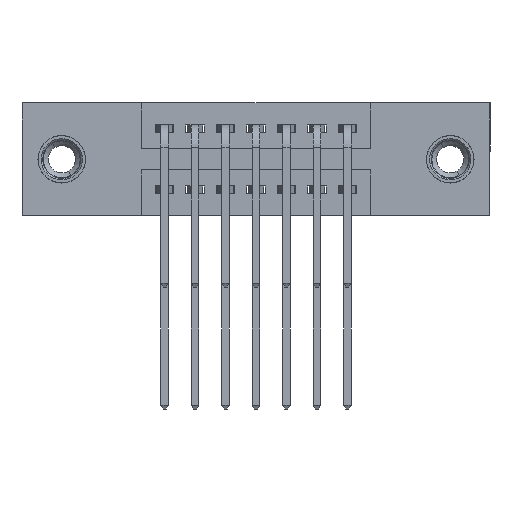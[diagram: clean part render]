
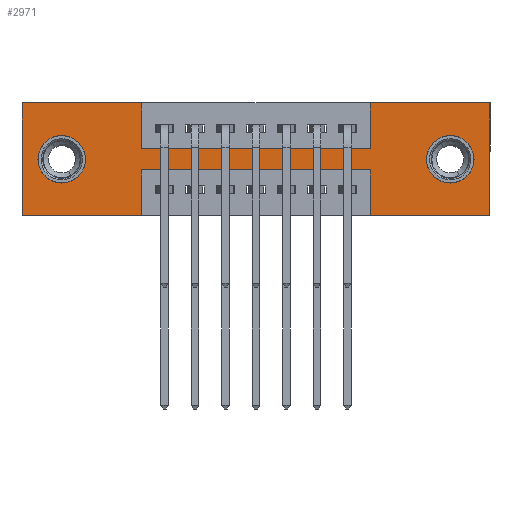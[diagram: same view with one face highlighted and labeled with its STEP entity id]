
A CAD part, front view. The second image highlights one B-rep face of the part: STEP entity #2971.
In plain terms, the highlighted planar face has unit normal (0, -1, 0).
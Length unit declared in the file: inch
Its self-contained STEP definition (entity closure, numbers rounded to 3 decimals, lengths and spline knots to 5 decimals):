
#73 = CARTESIAN_POINT ( 'NONE',  ( 1.535, 0., -0.37 ) ) ;
#83 = CIRCLE ( 'NONE', #9431, 0.078 ) ;
#284 = CARTESIAN_POINT ( 'NONE',  ( 0.13, 0., -0.185 ) ) ;
#466 = LINE ( 'NONE', #4444, #2477 ) ;
#517 = CARTESIAN_POINT ( 'NONE',  ( 0., 0., 0. ) ) ;
#733 = ORIENTED_EDGE ( 'NONE', *, *, #6720, .F. ) ;
#952 = LINE ( 'NONE', #956, #1924 ) ;
#956 = CARTESIAN_POINT ( 'NONE',  ( 1.1425, 0., 0. ) ) ;
#969 = VERTEX_POINT ( 'NONE', #12211 ) ;
#1108 = EDGE_CURVE ( 'NONE', #969, #10599, #4543, .T. ) ;
#1147 = LINE ( 'NONE', #5865, #10351 ) ;
#1169 = LINE ( 'NONE', #12165, #13202 ) ;
#1315 = ORIENTED_EDGE ( 'NONE', *, *, #10572, .F. ) ;
#1514 = DIRECTION ( 'NONE',  ( 0., 1., 0. ) ) ;
#1740 = DIRECTION ( 'NONE',  ( 0., 0., 1. ) ) ;
#1819 = ORIENTED_EDGE ( 'NONE', *, *, #13611, .T. ) ;
#1858 = VERTEX_POINT ( 'NONE', #15490 ) ;
#1884 = CARTESIAN_POINT ( 'NONE',  ( 1.405, 0., -0.263 ) ) ;
#1924 = VECTOR ( 'NONE', #2240, 39.37008 ) ;
#2062 = LINE ( 'NONE', #3148, #13703 ) ;
#2078 = LINE ( 'NONE', #15148, #12122 ) ;
#2105 = DIRECTION ( 'NONE',  ( 0., -1., 0. ) ) ;
#2240 = DIRECTION ( 'NONE',  ( 0., 0., 1. ) ) ;
#2336 = DIRECTION ( 'NONE',  ( -1., 0., 0. ) ) ;
#2477 = VECTOR ( 'NONE', #12230, 39.37008 ) ;
#2587 = VERTEX_POINT ( 'NONE', #8016 ) ;
#2615 = CARTESIAN_POINT ( 'NONE',  ( 1.1425, 0., -0.37 ) ) ;
#2679 = CIRCLE ( 'NONE', #10899, 0.078 ) ;
#2900 = ORIENTED_EDGE ( 'NONE', *, *, #11355, .F. ) ;
#2971 = ADVANCED_FACE ( 'NONE', ( #5885, #15959, #8110 ), #14921, .T. ) ;
#3127 = CARTESIAN_POINT ( 'NONE',  ( 0., 0., -0.37 ) ) ;
#3148 = CARTESIAN_POINT ( 'NONE',  ( 0.3925, 0., -0.22 ) ) ;
#3172 = ORIENTED_EDGE ( 'NONE', *, *, #3403, .F. ) ;
#3249 = ORIENTED_EDGE ( 'NONE', *, *, #10034, .T. ) ;
#3291 = DIRECTION ( 'NONE',  ( 0., 0., -1. ) ) ;
#3352 = CARTESIAN_POINT ( 'NONE',  ( 0.3925, 0., -0.37 ) ) ;
#3403 = EDGE_CURVE ( 'NONE', #8047, #969, #5868, .T. ) ;
#3492 = ORIENTED_EDGE ( 'NONE', *, *, #6524, .F. ) ;
#3503 = EDGE_CURVE ( 'NONE', #13259, #15265, #2062, .T. ) ;
#3588 = ORIENTED_EDGE ( 'NONE', *, *, #3503, .F. ) ;
#3594 = ORIENTED_EDGE ( 'NONE', *, *, #15354, .F. ) ;
#3632 = CARTESIAN_POINT ( 'NONE',  ( 1.405, 0., -0.185 ) ) ;
#3875 = AXIS2_PLACEMENT_3D ( 'NONE', #4564, #2105, #16044 ) ;
#4012 = EDGE_CURVE ( 'NONE', #14230, #12849, #14504, .T. ) ;
#4159 = EDGE_CURVE ( 'NONE', #4937, #5588, #1147, .T. ) ;
#4268 = CARTESIAN_POINT ( 'NONE',  ( 0.3925, 0., -0.15 ) ) ;
#4438 = EDGE_CURVE ( 'NONE', #15265, #9658, #6528, .T. ) ;
#4444 = CARTESIAN_POINT ( 'NONE',  ( 0., 0., 0. ) ) ;
#4543 = LINE ( 'NONE', #5618, #14598 ) ;
#4564 = CARTESIAN_POINT ( 'NONE',  ( 0., 0., -0.37 ) ) ;
#4937 = VERTEX_POINT ( 'NONE', #5871 ) ;
#5144 = EDGE_LOOP ( 'NONE', ( #3249, #5856 ) ) ;
#5428 = CARTESIAN_POINT ( 'NONE',  ( 0.3925, 0., -0.15 ) ) ;
#5588 = VERTEX_POINT ( 'NONE', #73 ) ;
#5618 = CARTESIAN_POINT ( 'NONE',  ( 0., 0., 0. ) ) ;
#5634 = DIRECTION ( 'NONE',  ( 1., 0., 0. ) ) ;
#5856 = ORIENTED_EDGE ( 'NONE', *, *, #15892, .T. ) ;
#5865 = CARTESIAN_POINT ( 'NONE',  ( 1.535, 0., 0. ) ) ;
#5868 = LINE ( 'NONE', #517, #9500 ) ;
#5871 = CARTESIAN_POINT ( 'NONE',  ( 1.535, 0., 0. ) ) ;
#5885 = FACE_BOUND ( 'NONE', #13947, .T. ) ;
#6087 = EDGE_CURVE ( 'NONE', #9594, #12605, #83, .T. ) ;
#6524 = EDGE_CURVE ( 'NONE', #7493, #4937, #466, .T. ) ;
#6528 = LINE ( 'NONE', #15635, #7151 ) ;
#6720 = EDGE_CURVE ( 'NONE', #9658, #8047, #2078, .T. ) ;
#6773 = DIRECTION ( 'NONE',  ( -1., 0., 0. ) ) ;
#7151 = VECTOR ( 'NONE', #14178, 39.37008 ) ;
#7493 = VERTEX_POINT ( 'NONE', #8682 ) ;
#7620 = LINE ( 'NONE', #14292, #11233 ) ;
#8008 = CARTESIAN_POINT ( 'NONE',  ( 0.13, 0., -0.185 ) ) ;
#8016 = CARTESIAN_POINT ( 'NONE',  ( 0.13, 0., -0.107 ) ) ;
#8047 = VERTEX_POINT ( 'NONE', #3127 ) ;
#8110 = FACE_OUTER_BOUND ( 'NONE', #15826, .T. ) ;
#8126 = DIRECTION ( 'NONE',  ( 0., 1., 0. ) ) ;
#8189 = DIRECTION ( 'NONE',  ( 0., 0., -1. ) ) ;
#8456 = DIRECTION ( 'NONE',  ( -1., 0., 0. ) ) ;
#8682 = CARTESIAN_POINT ( 'NONE',  ( 1.1425, 0., 0. ) ) ;
#8845 = CARTESIAN_POINT ( 'NONE',  ( 1.1425, 0., -0.22 ) ) ;
#9047 = DIRECTION ( 'NONE',  ( 0., 0., 1. ) ) ;
#9128 = CARTESIAN_POINT ( 'NONE',  ( 1.1425, 0., -0.37 ) ) ;
#9431 = AXIS2_PLACEMENT_3D ( 'NONE', #3632, #13858, #16614 ) ;
#9500 = VECTOR ( 'NONE', #13466, 39.37008 ) ;
#9594 = VERTEX_POINT ( 'NONE', #1884 ) ;
#9613 = ORIENTED_EDGE ( 'NONE', *, *, #4012, .F. ) ;
#9658 = VERTEX_POINT ( 'NONE', #3352 ) ;
#9926 = CARTESIAN_POINT ( 'NONE',  ( 1.405, 0., -0.107 ) ) ;
#10034 = EDGE_CURVE ( 'NONE', #2587, #1858, #11814, .T. ) ;
#10351 = VECTOR ( 'NONE', #3291, 39.37008 ) ;
#10512 = CARTESIAN_POINT ( 'NONE',  ( 1.1425, 0., -0.15 ) ) ;
#10572 = EDGE_CURVE ( 'NONE', #5588, #15701, #7620, .T. ) ;
#10599 = VERTEX_POINT ( 'NONE', #14350 ) ;
#10899 = AXIS2_PLACEMENT_3D ( 'NONE', #13092, #8126, #11932 ) ;
#11233 = VECTOR ( 'NONE', #6773, 39.37008 ) ;
#11244 = LINE ( 'NONE', #2615, #15656 ) ;
#11355 = EDGE_CURVE ( 'NONE', #12849, #7493, #952, .T. ) ;
#11562 = AXIS2_PLACEMENT_3D ( 'NONE', #284, #1514, #1740 ) ;
#11814 = CIRCLE ( 'NONE', #16455, 0.078 ) ;
#11928 = DIRECTION ( 'NONE',  ( 0., 1., 0. ) ) ;
#11932 = DIRECTION ( 'NONE',  ( 0., 0., -1. ) ) ;
#12011 = ORIENTED_EDGE ( 'NONE', *, *, #6087, .T. ) ;
#12122 = VECTOR ( 'NONE', #2336, 39.37008 ) ;
#12165 = CARTESIAN_POINT ( 'NONE',  ( 0.3925, 0., 0. ) ) ;
#12211 = CARTESIAN_POINT ( 'NONE',  ( 0., 0., 0. ) ) ;
#12230 = DIRECTION ( 'NONE',  ( 1., 0., 0. ) ) ;
#12605 = VERTEX_POINT ( 'NONE', #9926 ) ;
#12612 = ORIENTED_EDGE ( 'NONE', *, *, #15113, .F. ) ;
#12849 = VERTEX_POINT ( 'NONE', #10512 ) ;
#13053 = ORIENTED_EDGE ( 'NONE', *, *, #1108, .F. ) ;
#13092 = CARTESIAN_POINT ( 'NONE',  ( 1.405, 0., -0.185 ) ) ;
#13202 = VECTOR ( 'NONE', #8189, 39.37008 ) ;
#13259 = VERTEX_POINT ( 'NONE', #8845 ) ;
#13271 = DIRECTION ( 'NONE',  ( 1., 0., 0. ) ) ;
#13466 = DIRECTION ( 'NONE',  ( 0., 0., 1. ) ) ;
#13611 = EDGE_CURVE ( 'NONE', #12605, #9594, #2679, .T. ) ;
#13703 = VECTOR ( 'NONE', #8456, 39.37008 ) ;
#13858 = DIRECTION ( 'NONE',  ( 0., 1., 0. ) ) ;
#13947 = EDGE_LOOP ( 'NONE', ( #1819, #12011 ) ) ;
#14178 = DIRECTION ( 'NONE',  ( 0., 0., -1. ) ) ;
#14230 = VERTEX_POINT ( 'NONE', #5428 ) ;
#14279 = DIRECTION ( 'NONE',  ( 0., 0., 1. ) ) ;
#14292 = CARTESIAN_POINT ( 'NONE',  ( 0., 0., -0.37 ) ) ;
#14350 = CARTESIAN_POINT ( 'NONE',  ( 0.3925, 0., 0. ) ) ;
#14425 = CIRCLE ( 'NONE', #11562, 0.078 ) ;
#14487 = ORIENTED_EDGE ( 'NONE', *, *, #4159, .F. ) ;
#14504 = LINE ( 'NONE', #4268, #16321 ) ;
#14514 = CARTESIAN_POINT ( 'NONE',  ( 0.3925, 0., -0.22 ) ) ;
#14598 = VECTOR ( 'NONE', #5634, 39.37008 ) ;
#14921 = PLANE ( 'NONE',  #3875 ) ;
#15054 = ORIENTED_EDGE ( 'NONE', *, *, #4438, .F. ) ;
#15113 = EDGE_CURVE ( 'NONE', #15701, #13259, #11244, .T. ) ;
#15148 = CARTESIAN_POINT ( 'NONE',  ( 0., 0., -0.37 ) ) ;
#15265 = VERTEX_POINT ( 'NONE', #14514 ) ;
#15354 = EDGE_CURVE ( 'NONE', #10599, #14230, #1169, .T. ) ;
#15490 = CARTESIAN_POINT ( 'NONE',  ( 0.13, 0., -0.263 ) ) ;
#15635 = CARTESIAN_POINT ( 'NONE',  ( 0.3925, 0., -0.37 ) ) ;
#15656 = VECTOR ( 'NONE', #9047, 39.37008 ) ;
#15701 = VERTEX_POINT ( 'NONE', #9128 ) ;
#15826 = EDGE_LOOP ( 'NONE', ( #15054, #3588, #12612, #1315, #14487, #3492, #2900, #9613, #3594, #13053, #3172, #733 ) ) ;
#15892 = EDGE_CURVE ( 'NONE', #1858, #2587, #14425, .T. ) ;
#15959 = FACE_BOUND ( 'NONE', #5144, .T. ) ;
#16044 = DIRECTION ( 'NONE',  ( 0., 0., -1. ) ) ;
#16321 = VECTOR ( 'NONE', #13271, 39.37008 ) ;
#16455 = AXIS2_PLACEMENT_3D ( 'NONE', #8008, #11928, #14279 ) ;
#16614 = DIRECTION ( 'NONE',  ( 0., 0., -1. ) ) ;
